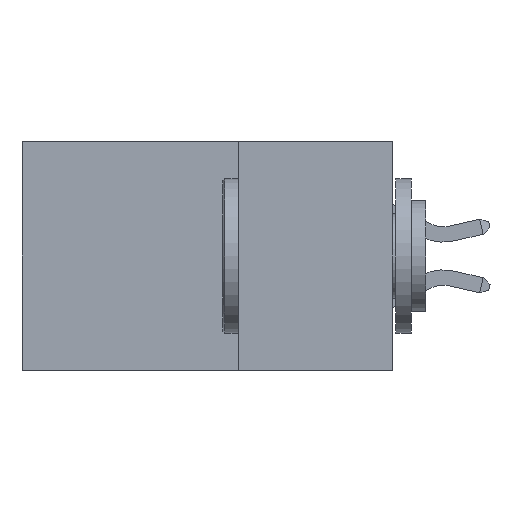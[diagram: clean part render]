
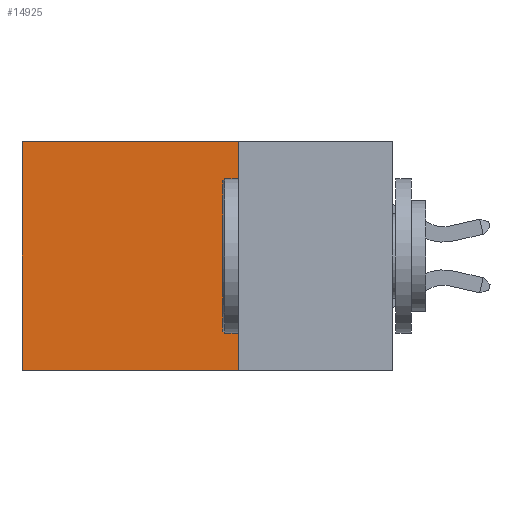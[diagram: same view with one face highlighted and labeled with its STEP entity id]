
A CAD part, left-side view. The second image highlights one B-rep face of the part: STEP entity #14925.
In plain terms, the highlighted planar face has unit normal (-1, 0, 0).
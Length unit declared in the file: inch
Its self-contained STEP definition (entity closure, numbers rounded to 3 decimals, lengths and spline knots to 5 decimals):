
#25 = EDGE_CURVE ( 'NONE', #5068, #4778, #16379, .T. ) ;
#629 = VECTOR ( 'NONE', #19581, 39.37008 ) ;
#1987 = FACE_OUTER_BOUND ( 'NONE', #3668, .T. ) ;
#2239 = VECTOR ( 'NONE', #15268, 39.37008 ) ;
#2694 = CARTESIAN_POINT ( 'NONE',  ( 0.2875, 0.25, 0. ) ) ;
#3668 = EDGE_LOOP ( 'NONE', ( #16086, #14602, #10311, #8164 ) ) ;
#3929 = AXIS2_PLACEMENT_3D ( 'NONE', #4884, #18619, #4961 ) ;
#4686 = LINE ( 'NONE', #16099, #629 ) ;
#4778 = VERTEX_POINT ( 'NONE', #6158 ) ;
#4884 = CARTESIAN_POINT ( 'NONE',  ( 0.2875, 0.25, 0. ) ) ;
#4961 = DIRECTION ( 'NONE',  ( 0., 0., -1. ) ) ;
#5068 = VERTEX_POINT ( 'NONE', #6951 ) ;
#6042 = DIRECTION ( 'NONE',  ( 0., 0., -1. ) ) ;
#6158 = CARTESIAN_POINT ( 'NONE',  ( 0.2875, 0.25, -0.37 ) ) ;
#6185 = EDGE_CURVE ( 'NONE', #5068, #22131, #11115, .T. ) ;
#6951 = CARTESIAN_POINT ( 'NONE',  ( 0.2875, 0.25, 0. ) ) ;
#7262 = EDGE_CURVE ( 'NONE', #4778, #14382, #4686, .T. ) ;
#8164 = ORIENTED_EDGE ( 'NONE', *, *, #6185, .T. ) ;
#10243 = CARTESIAN_POINT ( 'NONE',  ( 0.2875, 0.25, 0. ) ) ;
#10311 = ORIENTED_EDGE ( 'NONE', *, *, #25, .F. ) ;
#10734 = LINE ( 'NONE', #17741, #11565 ) ;
#11115 = LINE ( 'NONE', #2694, #16496 ) ;
#11565 = VECTOR ( 'NONE', #6042, 39.37008 ) ;
#14382 = VERTEX_POINT ( 'NONE', #15177 ) ;
#14602 = ORIENTED_EDGE ( 'NONE', *, *, #7262, .F. ) ;
#14925 = ADVANCED_FACE ( 'NONE', ( #1987 ), #18330, .F. ) ;
#15177 = CARTESIAN_POINT ( 'NONE',  ( 0.2875, 0.6, -0.37 ) ) ;
#15268 = DIRECTION ( 'NONE',  ( 0., 0., -1. ) ) ;
#15327 = EDGE_CURVE ( 'NONE', #22131, #14382, #10734, .T. ) ;
#16086 = ORIENTED_EDGE ( 'NONE', *, *, #15327, .T. ) ;
#16099 = CARTESIAN_POINT ( 'NONE',  ( 0.2875, 0.25, -0.37 ) ) ;
#16379 = LINE ( 'NONE', #10243, #2239 ) ;
#16496 = VECTOR ( 'NONE', #19805, 39.37008 ) ;
#17741 = CARTESIAN_POINT ( 'NONE',  ( 0.2875, 0.6, 0. ) ) ;
#18330 = PLANE ( 'NONE',  #3929 ) ;
#18619 = DIRECTION ( 'NONE',  ( 1., 0., 0. ) ) ;
#19054 = CARTESIAN_POINT ( 'NONE',  ( 0.2875, 0.6, 0. ) ) ;
#19581 = DIRECTION ( 'NONE',  ( 0., 1., 0. ) ) ;
#19805 = DIRECTION ( 'NONE',  ( 0., 1., 0. ) ) ;
#22131 = VERTEX_POINT ( 'NONE', #19054 ) ;
